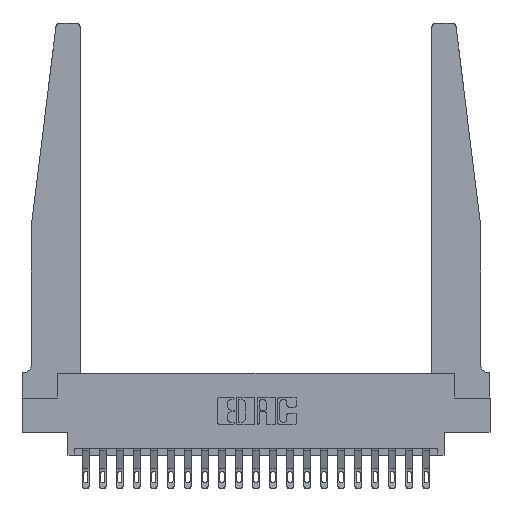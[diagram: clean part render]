
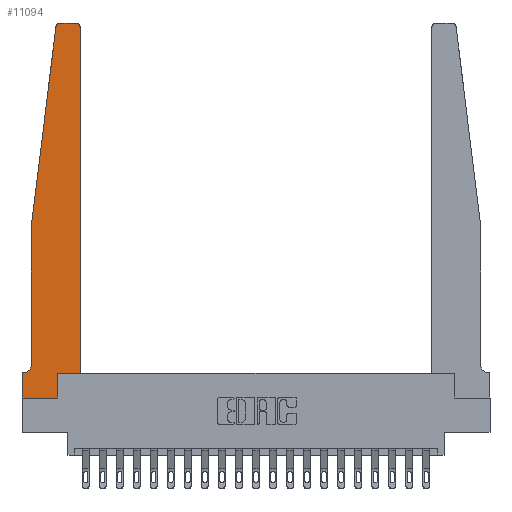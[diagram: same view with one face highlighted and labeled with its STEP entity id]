
A CAD part, top view. The second image highlights one B-rep face of the part: STEP entity #11094.
In plain terms, the highlighted planar face has unit normal (0, 0, 1).
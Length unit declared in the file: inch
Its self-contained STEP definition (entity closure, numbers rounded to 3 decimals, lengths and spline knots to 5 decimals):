
#193 = CARTESIAN_POINT ( 'NONE',  ( 0.015, 0.1875, 0.37 ) ) ;
#263 = CARTESIAN_POINT ( 'NONE',  ( 0., 0., 0.37 ) ) ;
#386 = DIRECTION ( 'NONE',  ( 1., 0., 0. ) ) ;
#510 = DIRECTION ( 'NONE',  ( 0., 1., 0. ) ) ;
#668 = LINE ( 'NONE', #3354, #4628 ) ;
#800 = CARTESIAN_POINT ( 'NONE',  ( 0.425, 0.18, 0.37 ) ) ;
#1165 = VERTEX_POINT ( 'NONE', #19545 ) ;
#1189 = LINE ( 'NONE', #18112, #13046 ) ;
#1190 = EDGE_CURVE ( 'NONE', #2771, #1338, #10760, .T. ) ;
#1338 = VERTEX_POINT ( 'NONE', #14970 ) ;
#1594 = ORIENTED_EDGE ( 'NONE', *, *, #14977, .T. ) ;
#1789 = VECTOR ( 'NONE', #9532, 39.37008 ) ;
#1812 = CARTESIAN_POINT ( 'NONE',  ( 0.27653, 2.72, 0.37 ) ) ;
#1915 = VERTEX_POINT ( 'NONE', #18344 ) ;
#1940 = VERTEX_POINT ( 'NONE', #18412 ) ;
#2109 = ORIENTED_EDGE ( 'NONE', *, *, #12686, .T. ) ;
#2289 = VERTEX_POINT ( 'NONE', #800 ) ;
#2398 = LINE ( 'NONE', #3505, #19787 ) ;
#2670 = CARTESIAN_POINT ( 'NONE',  ( 0., 0., 0.37 ) ) ;
#2713 = LINE ( 'NONE', #263, #7172 ) ;
#2771 = VERTEX_POINT ( 'NONE', #193 ) ;
#3082 = EDGE_CURVE ( 'NONE', #13827, #2771, #4901, .T. ) ;
#3086 = ORIENTED_EDGE ( 'NONE', *, *, #5253, .T. ) ;
#3353 = ORIENTED_EDGE ( 'NONE', *, *, #8836, .T. ) ;
#3354 = CARTESIAN_POINT ( 'NONE',  ( 0.25, 2.75, 0.37 ) ) ;
#3505 = CARTESIAN_POINT ( 'NONE',  ( 0.425, 0.18, 0.37 ) ) ;
#3532 = DIRECTION ( 'NONE',  ( 1., 0., 0. ) ) ;
#3665 = DIRECTION ( 'NONE',  ( 0., -1., 0. ) ) ;
#3810 = AXIS2_PLACEMENT_3D ( 'NONE', #1812, #13597, #3532 ) ;
#4158 = PLANE ( 'NONE',  #14851 ) ;
#4628 = VECTOR ( 'NONE', #15105, 39.37008 ) ;
#4638 = EDGE_CURVE ( 'NONE', #1338, #8548, #2713, .T. ) ;
#4901 = CIRCLE ( 'NONE', #17860, 0.05 ) ;
#5012 = CARTESIAN_POINT ( 'NONE',  ( 0., 0., 0.37 ) ) ;
#5253 = EDGE_CURVE ( 'NONE', #17591, #2289, #2398, .T. ) ;
#5600 = LINE ( 'NONE', #15567, #14531 ) ;
#6114 = ORIENTED_EDGE ( 'NONE', *, *, #9536, .T. ) ;
#6556 = VECTOR ( 'NONE', #21750, 39.37008 ) ;
#6643 = ORIENTED_EDGE ( 'NONE', *, *, #3082, .T. ) ;
#7049 = ORIENTED_EDGE ( 'NONE', *, *, #19069, .T. ) ;
#7172 = VECTOR ( 'NONE', #3665, 39.37008 ) ;
#8032 = DIRECTION ( 'NONE',  ( 0., -1., 0. ) ) ;
#8542 = VERTEX_POINT ( 'NONE', #12757 ) ;
#8548 = VERTEX_POINT ( 'NONE', #2670 ) ;
#8576 = VECTOR ( 'NONE', #510, 39.37008 ) ;
#8836 = EDGE_CURVE ( 'NONE', #8542, #17591, #12540, .T. ) ;
#8869 = DIRECTION ( 'NONE',  ( 0., 1., 0. ) ) ;
#8904 = CARTESIAN_POINT ( 'NONE',  ( 0.2605, 0.18, 0.37 ) ) ;
#9231 = DIRECTION ( 'NONE',  ( 1., 0., 0. ) ) ;
#9397 = DIRECTION ( 'NONE',  ( 0., 0., -1. ) ) ;
#9532 = DIRECTION ( 'NONE',  ( -1., 0., 0. ) ) ;
#9536 = EDGE_CURVE ( 'NONE', #1915, #1940, #668, .T. ) ;
#10365 = CARTESIAN_POINT ( 'NONE',  ( 0.065, 0.2375, 0.37 ) ) ;
#10477 = DIRECTION ( 'NONE',  ( 0., 0., 1. ) ) ;
#10760 = LINE ( 'NONE', #12852, #1789 ) ;
#10972 = ORIENTED_EDGE ( 'NONE', *, *, #12105, .T. ) ;
#11094 = ADVANCED_FACE ( 'NONE', ( #16628 ), #4158, .T. ) ;
#11569 = LINE ( 'NONE', #5012, #6556 ) ;
#12105 = EDGE_CURVE ( 'NONE', #8548, #8542, #11569, .T. ) ;
#12540 = LINE ( 'NONE', #8904, #8576 ) ;
#12686 = EDGE_CURVE ( 'NONE', #1165, #1915, #17333, .T. ) ;
#12757 = CARTESIAN_POINT ( 'NONE',  ( 0.2605, 0., 0.37 ) ) ;
#12852 = CARTESIAN_POINT ( 'NONE',  ( 0.065, 0.1875, 0.37 ) ) ;
#12977 = CIRCLE ( 'NONE', #3810, 0.03 ) ;
#12982 = ORIENTED_EDGE ( 'NONE', *, *, #1190, .T. ) ;
#13046 = VECTOR ( 'NONE', #8032, 39.37008 ) ;
#13597 = DIRECTION ( 'NONE',  ( 0., 0., 1. ) ) ;
#13827 = VERTEX_POINT ( 'NONE', #10365 ) ;
#14215 = LINE ( 'NONE', #19654, #18698 ) ;
#14266 = EDGE_LOOP ( 'NONE', ( #6114, #17117, #21644, #1594, #6643, #12982, #17255, #10972, #3353, #3086, #7049, #2109 ) ) ;
#14531 = VECTOR ( 'NONE', #8869, 39.37008 ) ;
#14851 = AXIS2_PLACEMENT_3D ( 'NONE', #15933, #19305, #9231 ) ;
#14970 = CARTESIAN_POINT ( 'NONE',  ( 0., 0.1875, 0.37 ) ) ;
#14977 = EDGE_CURVE ( 'NONE', #20267, #13827, #1189, .T. ) ;
#15105 = DIRECTION ( 'NONE',  ( -1., 0., 0. ) ) ;
#15567 = CARTESIAN_POINT ( 'NONE',  ( 0.425, 0.18, 0.37 ) ) ;
#15933 = CARTESIAN_POINT ( 'NONE',  ( 0., 0.1875, 0.37 ) ) ;
#16458 = EDGE_CURVE ( 'NONE', #1940, #17214, #12977, .T. ) ;
#16628 = FACE_OUTER_BOUND ( 'NONE', #14266, .T. ) ;
#17117 = ORIENTED_EDGE ( 'NONE', *, *, #16458, .T. ) ;
#17181 = CARTESIAN_POINT ( 'NONE',  ( 0.2605, 0.18, 0.37 ) ) ;
#17214 = VERTEX_POINT ( 'NONE', #19313 ) ;
#17255 = ORIENTED_EDGE ( 'NONE', *, *, #4638, .T. ) ;
#17333 = CIRCLE ( 'NONE', #17707, 0.03 ) ;
#17591 = VERTEX_POINT ( 'NONE', #17181 ) ;
#17707 = AXIS2_PLACEMENT_3D ( 'NONE', #20539, #10477, #386 ) ;
#17860 = AXIS2_PLACEMENT_3D ( 'NONE', #19473, #9397, #21163 ) ;
#18112 = CARTESIAN_POINT ( 'NONE',  ( 0.065, 1.25, 0.37 ) ) ;
#18344 = CARTESIAN_POINT ( 'NONE',  ( 0.395, 2.75, 0.37 ) ) ;
#18412 = CARTESIAN_POINT ( 'NONE',  ( 0.27653, 2.75, 0.37 ) ) ;
#18645 = DIRECTION ( 'NONE',  ( 1., 0., 0. ) ) ;
#18698 = VECTOR ( 'NONE', #21327, 39.37008 ) ;
#19069 = EDGE_CURVE ( 'NONE', #2289, #1165, #5600, .T. ) ;
#19305 = DIRECTION ( 'NONE',  ( 0., 0., 1. ) ) ;
#19313 = CARTESIAN_POINT ( 'NONE',  ( 0.24675, 2.72367, 0.37 ) ) ;
#19473 = CARTESIAN_POINT ( 'NONE',  ( 0.015, 0.2375, 0.37 ) ) ;
#19545 = CARTESIAN_POINT ( 'NONE',  ( 0.425, 2.72, 0.37 ) ) ;
#19654 = CARTESIAN_POINT ( 'NONE',  ( 0.065, 1.25, 0.37 ) ) ;
#19787 = VECTOR ( 'NONE', #18645, 39.37008 ) ;
#20267 = VERTEX_POINT ( 'NONE', #20881 ) ;
#20539 = CARTESIAN_POINT ( 'NONE',  ( 0.395, 2.72, 0.37 ) ) ;
#20816 = EDGE_CURVE ( 'NONE', #17214, #20267, #14215, .T. ) ;
#20881 = CARTESIAN_POINT ( 'NONE',  ( 0.065, 1.25, 0.37 ) ) ;
#21163 = DIRECTION ( 'NONE',  ( -1., 0., 0. ) ) ;
#21327 = DIRECTION ( 'NONE',  ( -0.122, -0.992, 0. ) ) ;
#21644 = ORIENTED_EDGE ( 'NONE', *, *, #20816, .T. ) ;
#21750 = DIRECTION ( 'NONE',  ( 1., 0., 0. ) ) ;
